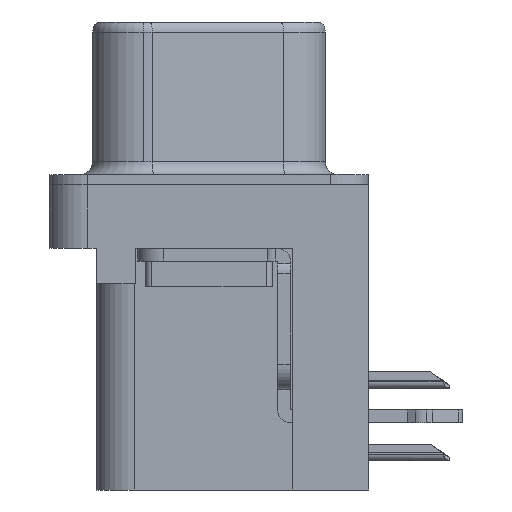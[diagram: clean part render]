
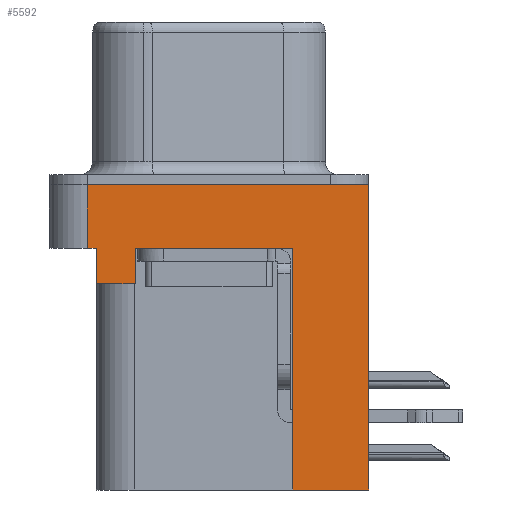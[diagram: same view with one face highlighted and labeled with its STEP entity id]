
A CAD part, left-side view. The second image highlights one B-rep face of the part: STEP entity #5592.
In plain terms, the highlighted planar face has unit normal (-1, 0, 0).
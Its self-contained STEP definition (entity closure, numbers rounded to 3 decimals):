
#32 = EDGE_CURVE ( 'NONE', #21825, #10603, #25082, .T. ) ;
#487 = CARTESIAN_POINT ( 'NONE',  ( -2.91, 2.895, -2.5 ) ) ;
#789 = CARTESIAN_POINT ( 'NONE',  ( -2.91, 2.895, -3.9 ) ) ;
#878 = LINE ( 'NONE', #4965, #22118 ) ;
#999 = EDGE_CURVE ( 'NONE', #4426, #4037, #2017, .T. ) ;
#1578 = VERTEX_POINT ( 'NONE', #20155 ) ;
#2017 = LINE ( 'NONE', #7672, #18336 ) ;
#2090 = EDGE_CURVE ( 'NONE', #10603, #24431, #878, .T. ) ;
#2255 = CARTESIAN_POINT ( 'NONE',  ( -2.91, -3.295, -2.5 ) ) ;
#2795 = LINE ( 'NONE', #9431, #13434 ) ;
#3108 = CARTESIAN_POINT ( 'NONE',  ( -2.91, -3.295, -12. ) ) ;
#3303 = AXIS2_PLACEMENT_3D ( 'NONE', #4024, #6185, #8310 ) ;
#3514 = ORIENTED_EDGE ( 'NONE', *, *, #20309, .F. ) ;
#3797 = EDGE_CURVE ( 'NONE', #9759, #24431, #2795, .T. ) ;
#4024 = CARTESIAN_POINT ( 'NONE',  ( -2.91, -6.275, -2.5 ) ) ;
#4037 = VERTEX_POINT ( 'NONE', #10854 ) ;
#4426 = VERTEX_POINT ( 'NONE', #13517 ) ;
#4562 = ORIENTED_EDGE ( 'NONE', *, *, #7054, .F. ) ;
#4646 = DIRECTION ( 'NONE',  ( 0., 0., 1. ) ) ;
#4676 = CARTESIAN_POINT ( 'NONE',  ( -2.91, -6.275, 0. ) ) ;
#4817 = VERTEX_POINT ( 'NONE', #13985 ) ;
#4965 = CARTESIAN_POINT ( 'NONE',  ( -2.91, -6.275, -2.5 ) ) ;
#5066 = EDGE_CURVE ( 'NONE', #24625, #24663, #9289, .T. ) ;
#5120 = ORIENTED_EDGE ( 'NONE', *, *, #9888, .F. ) ;
#5592 = ADVANCED_FACE ( 'NONE', ( #24274 ), #19298, .T. ) ;
#6044 = VECTOR ( 'NONE', #20585, 1000. ) ;
#6185 = DIRECTION ( 'NONE',  ( -1., 0., 0. ) ) ;
#6812 = DIRECTION ( 'NONE',  ( 0., -1., 0. ) ) ;
#7054 = EDGE_CURVE ( 'NONE', #4817, #1578, #24543, .T. ) ;
#7672 = CARTESIAN_POINT ( 'NONE',  ( -2.91, 4.425, -3.9 ) ) ;
#8310 = DIRECTION ( 'NONE',  ( 0., 0., 1. ) ) ;
#8368 = ORIENTED_EDGE ( 'NONE', *, *, #32, .T. ) ;
#8486 = CARTESIAN_POINT ( 'NONE',  ( -2.91, -3.295, -12. ) ) ;
#9289 = LINE ( 'NONE', #25215, #14264 ) ;
#9431 = CARTESIAN_POINT ( 'NONE',  ( -2.91, -3.295, -12. ) ) ;
#9759 = VERTEX_POINT ( 'NONE', #8486 ) ;
#9826 = CARTESIAN_POINT ( 'NONE',  ( -2.91, 4.425, -3.9 ) ) ;
#9888 = EDGE_CURVE ( 'NONE', #21825, #4426, #20359, .T. ) ;
#10086 = ORIENTED_EDGE ( 'NONE', *, *, #15251, .F. ) ;
#10384 = EDGE_CURVE ( 'NONE', #4817, #4037, #11323, .T. ) ;
#10603 = VERTEX_POINT ( 'NONE', #487 ) ;
#10854 = CARTESIAN_POINT ( 'NONE',  ( -2.91, 4.425, -2.5 ) ) ;
#11224 = VECTOR ( 'NONE', #26179, 1000. ) ;
#11323 = LINE ( 'NONE', #23737, #24320 ) ;
#11451 = DIRECTION ( 'NONE',  ( 0., 0., 1. ) ) ;
#11587 = DIRECTION ( 'NONE',  ( 0., 0., 1. ) ) ;
#11961 = DIRECTION ( 'NONE',  ( 0., 0., 1. ) ) ;
#12063 = DIRECTION ( 'NONE',  ( 0., 1., 0. ) ) ;
#13434 = VECTOR ( 'NONE', #11587, 1000. ) ;
#13517 = CARTESIAN_POINT ( 'NONE',  ( -2.91, 4.425, -3.9 ) ) ;
#13985 = CARTESIAN_POINT ( 'NONE',  ( -2.91, 4.775, -2.5 ) ) ;
#14079 = EDGE_LOOP ( 'NONE', ( #3514, #4562, #27115, #19003, #5120, #8368, #27372, #15637, #10086, #19227 ) ) ;
#14264 = VECTOR ( 'NONE', #23047, 1000. ) ;
#14547 = VECTOR ( 'NONE', #11451, 1000. ) ;
#15251 = EDGE_CURVE ( 'NONE', #24625, #9759, #16865, .T. ) ;
#15637 = ORIENTED_EDGE ( 'NONE', *, *, #3797, .F. ) ;
#16865 = LINE ( 'NONE', #3108, #11224 ) ;
#17603 = CARTESIAN_POINT ( 'NONE',  ( -2.91, 4.775, -2.5 ) ) ;
#18336 = VECTOR ( 'NONE', #11961, 1000. ) ;
#19003 = ORIENTED_EDGE ( 'NONE', *, *, #999, .F. ) ;
#19227 = ORIENTED_EDGE ( 'NONE', *, *, #5066, .T. ) ;
#19298 = PLANE ( 'NONE',  #3303 ) ;
#20155 = CARTESIAN_POINT ( 'NONE',  ( -2.91, 4.775, 0. ) ) ;
#20309 = EDGE_CURVE ( 'NONE', #1578, #24663, #23000, .T. ) ;
#20359 = LINE ( 'NONE', #9826, #26952 ) ;
#20490 = DIRECTION ( 'NONE',  ( 0., -1., 0. ) ) ;
#20585 = DIRECTION ( 'NONE',  ( 0., -1., 0. ) ) ;
#21572 = CARTESIAN_POINT ( 'NONE',  ( -2.91, 2.895, -3.9 ) ) ;
#21825 = VERTEX_POINT ( 'NONE', #789 ) ;
#22118 = VECTOR ( 'NONE', #20490, 1000. ) ;
#22136 = CARTESIAN_POINT ( 'NONE',  ( -2.91, -6.275, 0. ) ) ;
#23000 = LINE ( 'NONE', #22136, #6044 ) ;
#23047 = DIRECTION ( 'NONE',  ( 0., 0., 1. ) ) ;
#23737 = CARTESIAN_POINT ( 'NONE',  ( -2.91, -6.275, -2.5 ) ) ;
#24274 = FACE_OUTER_BOUND ( 'NONE', #14079, .T. ) ;
#24320 = VECTOR ( 'NONE', #6812, 1000. ) ;
#24431 = VERTEX_POINT ( 'NONE', #2255 ) ;
#24543 = LINE ( 'NONE', #17603, #14547 ) ;
#24625 = VERTEX_POINT ( 'NONE', #25890 ) ;
#24663 = VERTEX_POINT ( 'NONE', #4676 ) ;
#25082 = LINE ( 'NONE', #21572, #26742 ) ;
#25215 = CARTESIAN_POINT ( 'NONE',  ( -2.91, -6.275, -2.5 ) ) ;
#25890 = CARTESIAN_POINT ( 'NONE',  ( -2.91, -6.275, -12. ) ) ;
#26179 = DIRECTION ( 'NONE',  ( 0., 1., 0. ) ) ;
#26742 = VECTOR ( 'NONE', #4646, 1000. ) ;
#26952 = VECTOR ( 'NONE', #12063, 1000. ) ;
#27115 = ORIENTED_EDGE ( 'NONE', *, *, #10384, .T. ) ;
#27372 = ORIENTED_EDGE ( 'NONE', *, *, #2090, .T. ) ;
